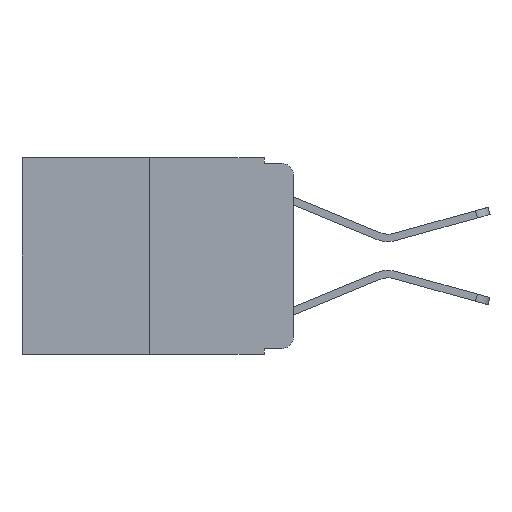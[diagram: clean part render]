
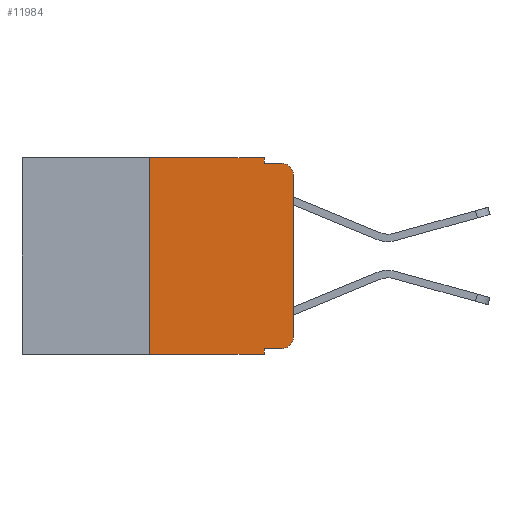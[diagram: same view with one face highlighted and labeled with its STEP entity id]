
A CAD part, left-side view. The second image highlights one B-rep face of the part: STEP entity #11984.
In plain terms, the highlighted planar face has unit normal (-1, 0, 0).
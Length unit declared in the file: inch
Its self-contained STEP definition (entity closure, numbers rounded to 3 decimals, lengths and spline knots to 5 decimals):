
#513 = DIRECTION ( 'NONE',  ( 0., 0., -1. ) ) ;
#644 = DIRECTION ( 'NONE',  ( 0., 0., -1. ) ) ;
#690 = DIRECTION ( 'NONE',  ( 0., 0., -1. ) ) ;
#817 = VERTEX_POINT ( 'NONE', #10503 ) ;
#969 = CIRCLE ( 'NONE', #19307, 0.02 ) ;
#1118 = PLANE ( 'NONE',  #6015 ) ;
#1423 = CIRCLE ( 'NONE', #20453, 0.02 ) ;
#1587 = CARTESIAN_POINT ( 'NONE',  ( 0., 0., -0.313 ) ) ;
#2303 = VERTEX_POINT ( 'NONE', #17324 ) ;
#2405 = LINE ( 'NONE', #16532, #3305 ) ;
#2616 = CARTESIAN_POINT ( 'NONE',  ( 0., 0.02, -0.03 ) ) ;
#2729 = ORIENTED_EDGE ( 'NONE', *, *, #4391, .F. ) ;
#3305 = VECTOR ( 'NONE', #20274, 39.37008 ) ;
#3942 = DIRECTION ( 'NONE',  ( 0., 0., 1. ) ) ;
#3988 = LINE ( 'NONE', #8880, #10557 ) ;
#4083 = EDGE_CURVE ( 'NONE', #10848, #17290, #10531, .T. ) ;
#4172 = VECTOR ( 'NONE', #12383, 39.37008 ) ;
#4182 = ORIENTED_EDGE ( 'NONE', *, *, #13322, .T. ) ;
#4391 = EDGE_CURVE ( 'NONE', #817, #19266, #11770, .T. ) ;
#4791 = CARTESIAN_POINT ( 'NONE',  ( 0., 0.051, -0.01 ) ) ;
#5106 = VECTOR ( 'NONE', #3942, 39.37008 ) ;
#5314 = CARTESIAN_POINT ( 'NONE',  ( 0., 0.051, 0. ) ) ;
#5815 = ORIENTED_EDGE ( 'NONE', *, *, #15393, .T. ) ;
#6015 = AXIS2_PLACEMENT_3D ( 'NONE', #9292, #10792, #19190 ) ;
#6780 = CARTESIAN_POINT ( 'NONE',  ( 0., 0.051, 0. ) ) ;
#7320 = VECTOR ( 'NONE', #513, 39.37008 ) ;
#7381 = EDGE_CURVE ( 'NONE', #17290, #19994, #10791, .T. ) ;
#7708 = ORIENTED_EDGE ( 'NONE', *, *, #20206, .T. ) ;
#8498 = LINE ( 'NONE', #5314, #19052 ) ;
#8720 = DIRECTION ( 'NONE',  ( 0., -1., 0. ) ) ;
#8880 = CARTESIAN_POINT ( 'NONE',  ( 0., 0.051, -0.01 ) ) ;
#9194 = DIRECTION ( 'NONE',  ( 0., -1., 0. ) ) ;
#9292 = CARTESIAN_POINT ( 'NONE',  ( 0., 0.473, 0. ) ) ;
#9423 = VECTOR ( 'NONE', #9194, 39.37008 ) ;
#9541 = ORIENTED_EDGE ( 'NONE', *, *, #7381, .F. ) ;
#9763 = ORIENTED_EDGE ( 'NONE', *, *, #18993, .F. ) ;
#9997 = VERTEX_POINT ( 'NONE', #1587 ) ;
#10282 = ORIENTED_EDGE ( 'NONE', *, *, #17014, .F. ) ;
#10503 = CARTESIAN_POINT ( 'NONE',  ( 0., 0.051, -0.333 ) ) ;
#10531 = LINE ( 'NONE', #12129, #5106 ) ;
#10557 = VECTOR ( 'NONE', #16535, 39.37008 ) ;
#10630 = DIRECTION ( 'NONE',  ( -1., 0., 0. ) ) ;
#10791 = LINE ( 'NONE', #18658, #4172 ) ;
#10792 = DIRECTION ( 'NONE',  ( 1., 0., 0. ) ) ;
#10848 = VERTEX_POINT ( 'NONE', #12916 ) ;
#11354 = CARTESIAN_POINT ( 'NONE',  ( 0., 0.051, -0.343 ) ) ;
#11770 = LINE ( 'NONE', #6780, #7320 ) ;
#11886 = EDGE_CURVE ( 'NONE', #9997, #2303, #2405, .T. ) ;
#11984 = ADVANCED_FACE ( 'NONE', ( #14207 ), #1118, .F. ) ;
#12129 = CARTESIAN_POINT ( 'NONE',  ( 0., 0.25, 0. ) ) ;
#12383 = DIRECTION ( 'NONE',  ( 0., -1., 0. ) ) ;
#12916 = CARTESIAN_POINT ( 'NONE',  ( 0., 0.25, -0.343 ) ) ;
#13117 = CARTESIAN_POINT ( 'NONE',  ( 0., 0.25, 0. ) ) ;
#13322 = EDGE_CURVE ( 'NONE', #817, #19841, #14209, .T. ) ;
#13336 = VERTEX_POINT ( 'NONE', #19704 ) ;
#13945 = DIRECTION ( 'NONE',  ( 0., 0., -1. ) ) ;
#14142 = EDGE_CURVE ( 'NONE', #19841, #9997, #969, .T. ) ;
#14207 = FACE_OUTER_BOUND ( 'NONE', #16147, .T. ) ;
#14209 = LINE ( 'NONE', #20697, #9423 ) ;
#14934 = CARTESIAN_POINT ( 'NONE',  ( 0., 0.051, 0. ) ) ;
#15393 = EDGE_CURVE ( 'NONE', #10848, #19266, #18614, .T. ) ;
#16147 = EDGE_LOOP ( 'NONE', ( #19256, #7708, #10282, #9763, #9541, #18612, #5815, #2729, #4182, #16692 ) ) ;
#16532 = CARTESIAN_POINT ( 'NONE',  ( 0., 0., 0. ) ) ;
#16535 = DIRECTION ( 'NONE',  ( 0., -1., 0. ) ) ;
#16692 = ORIENTED_EDGE ( 'NONE', *, *, #14142, .T. ) ;
#17014 = EDGE_CURVE ( 'NONE', #17695, #13336, #3988, .T. ) ;
#17031 = CARTESIAN_POINT ( 'NONE',  ( 0., 0.473, -0.343 ) ) ;
#17129 = CARTESIAN_POINT ( 'NONE',  ( 0., 0.02, -0.313 ) ) ;
#17290 = VERTEX_POINT ( 'NONE', #13117 ) ;
#17324 = CARTESIAN_POINT ( 'NONE',  ( 0., 0., -0.03 ) ) ;
#17695 = VERTEX_POINT ( 'NONE', #4791 ) ;
#18612 = ORIENTED_EDGE ( 'NONE', *, *, #4083, .F. ) ;
#18614 = LINE ( 'NONE', #17031, #20713 ) ;
#18658 = CARTESIAN_POINT ( 'NONE',  ( 0., 0.473, 0. ) ) ;
#18993 = EDGE_CURVE ( 'NONE', #19994, #17695, #8498, .T. ) ;
#19052 = VECTOR ( 'NONE', #644, 39.37008 ) ;
#19190 = DIRECTION ( 'NONE',  ( 0., 0., -1. ) ) ;
#19256 = ORIENTED_EDGE ( 'NONE', *, *, #11886, .T. ) ;
#19266 = VERTEX_POINT ( 'NONE', #11354 ) ;
#19307 = AXIS2_PLACEMENT_3D ( 'NONE', #17129, #10630, #13945 ) ;
#19704 = CARTESIAN_POINT ( 'NONE',  ( 0., 0.02, -0.01 ) ) ;
#19841 = VERTEX_POINT ( 'NONE', #20826 ) ;
#19994 = VERTEX_POINT ( 'NONE', #14934 ) ;
#20052 = DIRECTION ( 'NONE',  ( -1., 0., 0. ) ) ;
#20206 = EDGE_CURVE ( 'NONE', #2303, #13336, #1423, .T. ) ;
#20274 = DIRECTION ( 'NONE',  ( 0., 0., 1. ) ) ;
#20453 = AXIS2_PLACEMENT_3D ( 'NONE', #2616, #20052, #690 ) ;
#20697 = CARTESIAN_POINT ( 'NONE',  ( 0., 0.051, -0.333 ) ) ;
#20713 = VECTOR ( 'NONE', #8720, 39.37008 ) ;
#20826 = CARTESIAN_POINT ( 'NONE',  ( 0., 0.02, -0.333 ) ) ;
